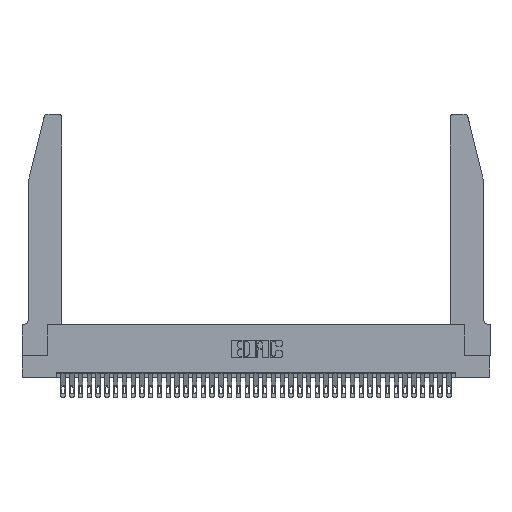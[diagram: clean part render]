
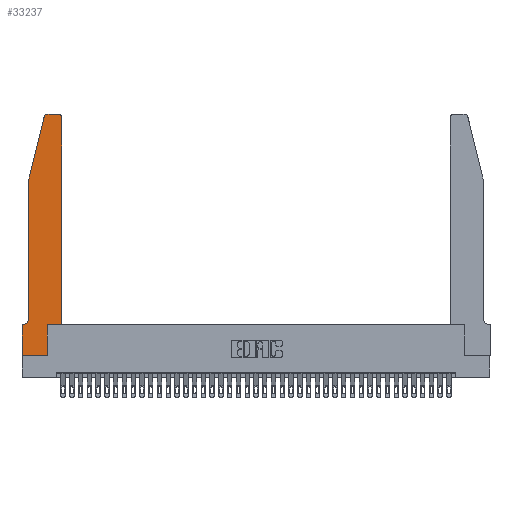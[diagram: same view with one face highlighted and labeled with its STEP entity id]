
A CAD part, top view. The second image highlights one B-rep face of the part: STEP entity #33237.
In plain terms, the highlighted planar face has unit normal (0, 0, 1).
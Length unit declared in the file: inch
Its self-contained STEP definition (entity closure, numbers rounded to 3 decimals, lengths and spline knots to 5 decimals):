
#178 = CARTESIAN_POINT ( 'NONE',  ( 0.0755, 2., 0.37 ) ) ;
#498 = CARTESIAN_POINT ( 'NONE',  ( 0., 0., 0.37 ) ) ;
#2696 = CARTESIAN_POINT ( 'NONE',  ( 0.4205, 2.72, 0.37 ) ) ;
#2699 = EDGE_CURVE ( 'NONE', #33940, #37736, #36128, .T. ) ;
#2744 = VERTEX_POINT ( 'NONE', #10843 ) ;
#3032 = LINE ( 'NONE', #7244, #26723 ) ;
#3250 = ORIENTED_EDGE ( 'NONE', *, *, #4560, .T. ) ;
#3335 = EDGE_CURVE ( 'NONE', #34758, #9274, #7825, .T. ) ;
#4337 = LINE ( 'NONE', #498, #35127 ) ;
#4531 = CARTESIAN_POINT ( 'NONE',  ( 0., 0.35, 0.37 ) ) ;
#4560 = EDGE_CURVE ( 'NONE', #29828, #20485, #3032, .T. ) ;
#4666 = DIRECTION ( 'NONE',  ( 1., 0., 0. ) ) ;
#4701 = DIRECTION ( 'NONE',  ( 0., 1., 0. ) ) ;
#5892 = DIRECTION ( 'NONE',  ( 1., 0., 0. ) ) ;
#6119 = VERTEX_POINT ( 'NONE', #29661 ) ;
#6577 = DIRECTION ( 'NONE',  ( 1., 0., 0. ) ) ;
#6882 = VECTOR ( 'NONE', #4701, 39.37008 ) ;
#7244 = CARTESIAN_POINT ( 'NONE',  ( 0.0755, 2., 0.37 ) ) ;
#7254 = ORIENTED_EDGE ( 'NONE', *, *, #39260, .T. ) ;
#7445 = VERTEX_POINT ( 'NONE', #8558 ) ;
#7825 = LINE ( 'NONE', #31850, #15147 ) ;
#7885 = LINE ( 'NONE', #38702, #28513 ) ;
#8558 = CARTESIAN_POINT ( 'NONE',  ( 0.284, 2.75, 0.37 ) ) ;
#9274 = VERTEX_POINT ( 'NONE', #18633 ) ;
#9751 = ORIENTED_EDGE ( 'NONE', *, *, #27638, .T. ) ;
#10108 = VERTEX_POINT ( 'NONE', #16525 ) ;
#10332 = DIRECTION ( 'NONE',  ( 0., 0., -1. ) ) ;
#10627 = DIRECTION ( 'NONE',  ( 0., -1., 0. ) ) ;
#10708 = DIRECTION ( 'NONE',  ( 0., 1., 0. ) ) ;
#10843 = CARTESIAN_POINT ( 'NONE',  ( 0.0755, 0.42, 0.37 ) ) ;
#11194 = ORIENTED_EDGE ( 'NONE', *, *, #13559, .T. ) ;
#11679 = CARTESIAN_POINT ( 'NONE',  ( 0.2865, 0., 0.37 ) ) ;
#12065 = VERTEX_POINT ( 'NONE', #33806 ) ;
#12081 = DIRECTION ( 'NONE',  ( 0., 0., 1. ) ) ;
#12330 = CARTESIAN_POINT ( 'NONE',  ( 0.0755, 0.35, 0.37 ) ) ;
#12476 = EDGE_CURVE ( 'NONE', #26521, #6119, #15205, .T. ) ;
#12536 = EDGE_CURVE ( 'NONE', #10108, #7445, #7885, .T. ) ;
#12807 = EDGE_CURVE ( 'NONE', #9274, #33940, #4337, .T. ) ;
#13148 = ORIENTED_EDGE ( 'NONE', *, *, #17829, .T. ) ;
#13559 = EDGE_CURVE ( 'NONE', #2744, #12065, #18486, .T. ) ;
#13796 = LINE ( 'NONE', #35907, #29037 ) ;
#14100 = ORIENTED_EDGE ( 'NONE', *, *, #3335, .T. ) ;
#15145 = CARTESIAN_POINT ( 'NONE',  ( 0., 0.35, 0.37 ) ) ;
#15147 = VECTOR ( 'NONE', #10627, 39.37008 ) ;
#15205 = LINE ( 'NONE', #26315, #6882 ) ;
#15479 = CIRCLE ( 'NONE', #17979, 0.03 ) ;
#15779 = VECTOR ( 'NONE', #6577, 39.37008 ) ;
#16525 = CARTESIAN_POINT ( 'NONE',  ( 0.4205, 2.75, 0.37 ) ) ;
#16617 = DIRECTION ( 'NONE',  ( -0.239, -0.971, 0. ) ) ;
#16701 = FACE_OUTER_BOUND ( 'NONE', #38522, .T. ) ;
#17117 = PLANE ( 'NONE',  #38000 ) ;
#17829 = EDGE_CURVE ( 'NONE', #12065, #34758, #37441, .T. ) ;
#17979 = AXIS2_PLACEMENT_3D ( 'NONE', #30338, #12081, #33414 ) ;
#18486 = CIRCLE ( 'NONE', #39881, 0.07 ) ;
#18633 = CARTESIAN_POINT ( 'NONE',  ( 0., 0., 0.37 ) ) ;
#20485 = VERTEX_POINT ( 'NONE', #178 ) ;
#20777 = DIRECTION ( 'NONE',  ( 0., -1., 0. ) ) ;
#20846 = ORIENTED_EDGE ( 'NONE', *, *, #25857, .T. ) ;
#22202 = ORIENTED_EDGE ( 'NONE', *, *, #12536, .T. ) ;
#23221 = DIRECTION ( 'NONE',  ( 0., 0., 1. ) ) ;
#24365 = DIRECTION ( 'NONE',  ( 0., 0., 1. ) ) ;
#25020 = CARTESIAN_POINT ( 'NONE',  ( 0.4505, 0.35, 0.37 ) ) ;
#25070 = ORIENTED_EDGE ( 'NONE', *, *, #2699, .T. ) ;
#25349 = AXIS2_PLACEMENT_3D ( 'NONE', #2696, #24365, #5892 ) ;
#25377 = DIRECTION ( 'NONE',  ( 1., 0., 0. ) ) ;
#25857 = EDGE_CURVE ( 'NONE', #6119, #10108, #38696, .T. ) ;
#26010 = CARTESIAN_POINT ( 'NONE',  ( 0.2865, 0.35, 0.37 ) ) ;
#26315 = CARTESIAN_POINT ( 'NONE',  ( 0.4505, 0.35, 0.37 ) ) ;
#26521 = VERTEX_POINT ( 'NONE', #33927 ) ;
#26723 = VECTOR ( 'NONE', #16617, 39.37008 ) ;
#27418 = VECTOR ( 'NONE', #36702, 39.37008 ) ;
#27638 = EDGE_CURVE ( 'NONE', #37736, #26521, #30975, .T. ) ;
#28513 = VECTOR ( 'NONE', #29631, 39.37008 ) ;
#28652 = CARTESIAN_POINT ( 'NONE',  ( 0.0055, 0.42, 0.37 ) ) ;
#28976 = VECTOR ( 'NONE', #10708, 39.37008 ) ;
#28999 = CARTESIAN_POINT ( 'NONE',  ( 0.2865, 0.35, 0.37 ) ) ;
#29037 = VECTOR ( 'NONE', #20777, 39.37008 ) ;
#29475 = CARTESIAN_POINT ( 'NONE',  ( 0.25487, 2.72718, 0.37 ) ) ;
#29631 = DIRECTION ( 'NONE',  ( -1., 0., 0. ) ) ;
#29661 = CARTESIAN_POINT ( 'NONE',  ( 0.4505, 2.72, 0.37 ) ) ;
#29828 = VERTEX_POINT ( 'NONE', #29475 ) ;
#30338 = CARTESIAN_POINT ( 'NONE',  ( 0.284, 2.72, 0.37 ) ) ;
#30975 = LINE ( 'NONE', #25020, #15779 ) ;
#31241 = ORIENTED_EDGE ( 'NONE', *, *, #12807, .T. ) ;
#31708 = DIRECTION ( 'NONE',  ( -1., 0., 0. ) ) ;
#31850 = CARTESIAN_POINT ( 'NONE',  ( 0., 0., 0.37 ) ) ;
#33237 = ADVANCED_FACE ( 'NONE', ( #16701 ), #17117, .T. ) ;
#33414 = DIRECTION ( 'NONE',  ( 1., 0., 0. ) ) ;
#33806 = CARTESIAN_POINT ( 'NONE',  ( 0.0055, 0.35, 0.37 ) ) ;
#33927 = CARTESIAN_POINT ( 'NONE',  ( 0.4505, 0.35, 0.37 ) ) ;
#33940 = VERTEX_POINT ( 'NONE', #11679 ) ;
#34758 = VERTEX_POINT ( 'NONE', #15145 ) ;
#35017 = ORIENTED_EDGE ( 'NONE', *, *, #36720, .T. ) ;
#35055 = ORIENTED_EDGE ( 'NONE', *, *, #12476, .T. ) ;
#35127 = VECTOR ( 'NONE', #25377, 39.37008 ) ;
#35907 = CARTESIAN_POINT ( 'NONE',  ( 0.0755, 2., 0.37 ) ) ;
#36128 = LINE ( 'NONE', #28999, #28976 ) ;
#36702 = DIRECTION ( 'NONE',  ( -1., 0., 0. ) ) ;
#36720 = EDGE_CURVE ( 'NONE', #7445, #29828, #15479, .T. ) ;
#37441 = LINE ( 'NONE', #12330, #27418 ) ;
#37736 = VERTEX_POINT ( 'NONE', #26010 ) ;
#38000 = AXIS2_PLACEMENT_3D ( 'NONE', #4531, #23221, #4666 ) ;
#38522 = EDGE_LOOP ( 'NONE', ( #22202, #35017, #3250, #7254, #11194, #13148, #14100, #31241, #25070, #9751, #35055, #20846 ) ) ;
#38696 = CIRCLE ( 'NONE', #25349, 0.03 ) ;
#38702 = CARTESIAN_POINT ( 'NONE',  ( 0.2605, 2.75, 0.37 ) ) ;
#39260 = EDGE_CURVE ( 'NONE', #20485, #2744, #13796, .T. ) ;
#39881 = AXIS2_PLACEMENT_3D ( 'NONE', #28652, #10332, #31708 ) ;
